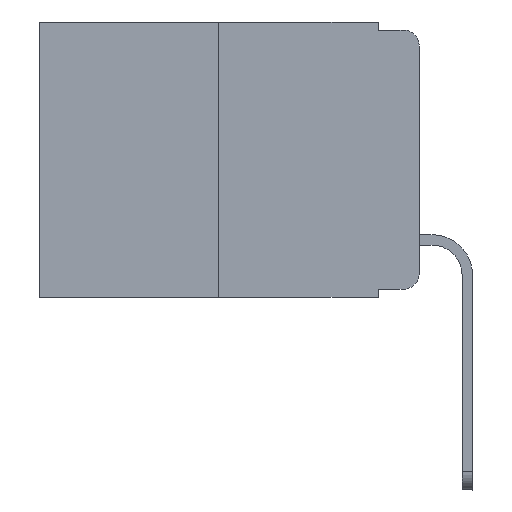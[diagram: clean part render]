
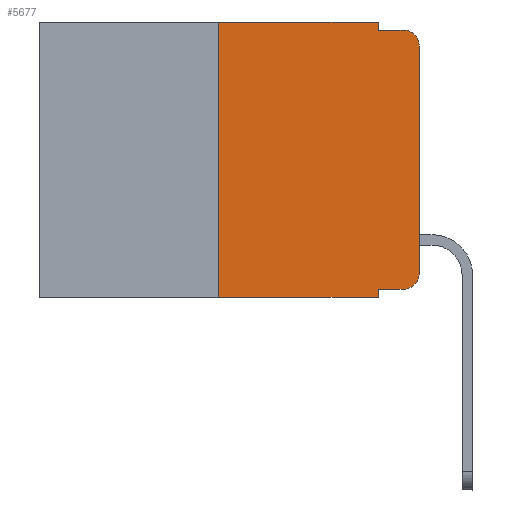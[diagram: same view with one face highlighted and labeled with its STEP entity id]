
A CAD part, left-side view. The second image highlights one B-rep face of the part: STEP entity #5677.
In plain terms, the highlighted planar face has unit normal (-1, 0, 0).
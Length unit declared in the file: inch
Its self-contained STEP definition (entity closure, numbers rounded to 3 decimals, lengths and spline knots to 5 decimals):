
#229 = EDGE_CURVE ( 'NONE', #13039, #11638, #12042, .T. ) ;
#322 = DIRECTION ( 'NONE',  ( -1., 0., 0. ) ) ;
#457 = ORIENTED_EDGE ( 'NONE', *, *, #5228, .T. ) ;
#520 = CARTESIAN_POINT ( 'NONE',  ( 0., 0.02, -0.03 ) ) ;
#587 = DIRECTION ( 'NONE',  ( 0., 0., -1. ) ) ;
#609 = LINE ( 'NONE', #13152, #14954 ) ;
#783 = LINE ( 'NONE', #6575, #14129 ) ;
#885 = PLANE ( 'NONE',  #15888 ) ;
#991 = CARTESIAN_POINT ( 'NONE',  ( 0., 0.473, 0. ) ) ;
#1045 = ORIENTED_EDGE ( 'NONE', *, *, #14758, .F. ) ;
#1281 = CARTESIAN_POINT ( 'NONE',  ( 0., 0.25, 0. ) ) ;
#1358 = CARTESIAN_POINT ( 'NONE',  ( 0., 0.051, 0. ) ) ;
#1618 = EDGE_CURVE ( 'NONE', #14833, #5186, #609, .T. ) ;
#1847 = DIRECTION ( 'NONE',  ( 0., -1., 0. ) ) ;
#1994 = EDGE_CURVE ( 'NONE', #4367, #3396, #9498, .T. ) ;
#2181 = VECTOR ( 'NONE', #8566, 39.37008 ) ;
#2862 = CARTESIAN_POINT ( 'NONE',  ( 0., 0.051, 0. ) ) ;
#2923 = ORIENTED_EDGE ( 'NONE', *, *, #1618, .T. ) ;
#3396 = VERTEX_POINT ( 'NONE', #14422 ) ;
#3688 = DIRECTION ( 'NONE',  ( 0., 0., 1. ) ) ;
#4367 = VERTEX_POINT ( 'NONE', #7631 ) ;
#4495 = ORIENTED_EDGE ( 'NONE', *, *, #16707, .F. ) ;
#4543 = DIRECTION ( 'NONE',  ( 0., 0., -1. ) ) ;
#4610 = LINE ( 'NONE', #10313, #14127 ) ;
#4735 = DIRECTION ( 'NONE',  ( 0., 0., -1. ) ) ;
#4755 = CARTESIAN_POINT ( 'NONE',  ( 0., 0.051, -0.01 ) ) ;
#4833 = DIRECTION ( 'NONE',  ( 1., 0., 0. ) ) ;
#4874 = AXIS2_PLACEMENT_3D ( 'NONE', #520, #322, #4735 ) ;
#5066 = VECTOR ( 'NONE', #1847, 39.37008 ) ;
#5182 = VERTEX_POINT ( 'NONE', #6459 ) ;
#5186 = VERTEX_POINT ( 'NONE', #12436 ) ;
#5228 = EDGE_CURVE ( 'NONE', #3396, #13039, #5246, .T. ) ;
#5246 = LINE ( 'NONE', #16439, #10789 ) ;
#5676 = LINE ( 'NONE', #14276, #10801 ) ;
#5677 = ADVANCED_FACE ( 'NONE', ( #13703 ), #885, .F. ) ;
#5860 = EDGE_LOOP ( 'NONE', ( #457, #13875, #8158, #10997, #18421, #4495, #2923, #1045, #13607, #15305 ) ) ;
#6354 = LINE ( 'NONE', #4755, #5066 ) ;
#6417 = EDGE_CURVE ( 'NONE', #5182, #4367, #8603, .T. ) ;
#6459 = CARTESIAN_POINT ( 'NONE',  ( 0., 0.051, -0.333 ) ) ;
#6575 = CARTESIAN_POINT ( 'NONE',  ( 0., 0.25, 0. ) ) ;
#7534 = DIRECTION ( 'NONE',  ( 0., -1., 0. ) ) ;
#7631 = CARTESIAN_POINT ( 'NONE',  ( 0., 0.02, -0.333 ) ) ;
#8158 = ORIENTED_EDGE ( 'NONE', *, *, #15660, .F. ) ;
#8566 = DIRECTION ( 'NONE',  ( 0., 0., -1. ) ) ;
#8603 = LINE ( 'NONE', #14314, #16793 ) ;
#8883 = CARTESIAN_POINT ( 'NONE',  ( 0., 0., -0.03 ) ) ;
#9013 = DIRECTION ( 'NONE',  ( -1., 0., 0. ) ) ;
#9498 = CIRCLE ( 'NONE', #15481, 0.02 ) ;
#10313 = CARTESIAN_POINT ( 'NONE',  ( 0., 0.473, 0. ) ) ;
#10533 = DIRECTION ( 'NONE',  ( 0., 0., -1. ) ) ;
#10789 = VECTOR ( 'NONE', #13553, 39.37008 ) ;
#10801 = VECTOR ( 'NONE', #4543, 39.37008 ) ;
#10997 = ORIENTED_EDGE ( 'NONE', *, *, #13948, .F. ) ;
#11638 = VERTEX_POINT ( 'NONE', #18158 ) ;
#12042 = CIRCLE ( 'NONE', #4874, 0.02 ) ;
#12436 = CARTESIAN_POINT ( 'NONE',  ( 0., 0.051, -0.343 ) ) ;
#12542 = DIRECTION ( 'NONE',  ( 0., -1., 0. ) ) ;
#13039 = VERTEX_POINT ( 'NONE', #8883 ) ;
#13152 = CARTESIAN_POINT ( 'NONE',  ( 0., 0.473, -0.343 ) ) ;
#13241 = CARTESIAN_POINT ( 'NONE',  ( 0., 0.25, -0.343 ) ) ;
#13404 = CARTESIAN_POINT ( 'NONE',  ( 0., 0.02, -0.313 ) ) ;
#13553 = DIRECTION ( 'NONE',  ( 0., 0., 1. ) ) ;
#13607 = ORIENTED_EDGE ( 'NONE', *, *, #6417, .T. ) ;
#13703 = FACE_OUTER_BOUND ( 'NONE', #5860, .T. ) ;
#13875 = ORIENTED_EDGE ( 'NONE', *, *, #229, .T. ) ;
#13948 = EDGE_CURVE ( 'NONE', #16369, #15425, #5676, .T. ) ;
#14127 = VECTOR ( 'NONE', #16190, 39.37008 ) ;
#14129 = VECTOR ( 'NONE', #3688, 39.37008 ) ;
#14276 = CARTESIAN_POINT ( 'NONE',  ( 0., 0.051, 0. ) ) ;
#14314 = CARTESIAN_POINT ( 'NONE',  ( 0., 0.051, -0.333 ) ) ;
#14422 = CARTESIAN_POINT ( 'NONE',  ( 0., 0., -0.313 ) ) ;
#14676 = VERTEX_POINT ( 'NONE', #1281 ) ;
#14758 = EDGE_CURVE ( 'NONE', #5182, #5186, #15691, .T. ) ;
#14833 = VERTEX_POINT ( 'NONE', #13241 ) ;
#14954 = VECTOR ( 'NONE', #7534, 39.37008 ) ;
#15305 = ORIENTED_EDGE ( 'NONE', *, *, #1994, .T. ) ;
#15425 = VERTEX_POINT ( 'NONE', #18144 ) ;
#15481 = AXIS2_PLACEMENT_3D ( 'NONE', #13404, #9013, #587 ) ;
#15660 = EDGE_CURVE ( 'NONE', #15425, #11638, #6354, .T. ) ;
#15691 = LINE ( 'NONE', #2862, #2181 ) ;
#15888 = AXIS2_PLACEMENT_3D ( 'NONE', #991, #4833, #10533 ) ;
#16190 = DIRECTION ( 'NONE',  ( 0., -1., 0. ) ) ;
#16369 = VERTEX_POINT ( 'NONE', #1358 ) ;
#16439 = CARTESIAN_POINT ( 'NONE',  ( 0., 0., 0. ) ) ;
#16707 = EDGE_CURVE ( 'NONE', #14833, #14676, #783, .T. ) ;
#16793 = VECTOR ( 'NONE', #12542, 39.37008 ) ;
#18144 = CARTESIAN_POINT ( 'NONE',  ( 0., 0.051, -0.01 ) ) ;
#18158 = CARTESIAN_POINT ( 'NONE',  ( 0., 0.02, -0.01 ) ) ;
#18387 = EDGE_CURVE ( 'NONE', #14676, #16369, #4610, .T. ) ;
#18421 = ORIENTED_EDGE ( 'NONE', *, *, #18387, .F. ) ;
